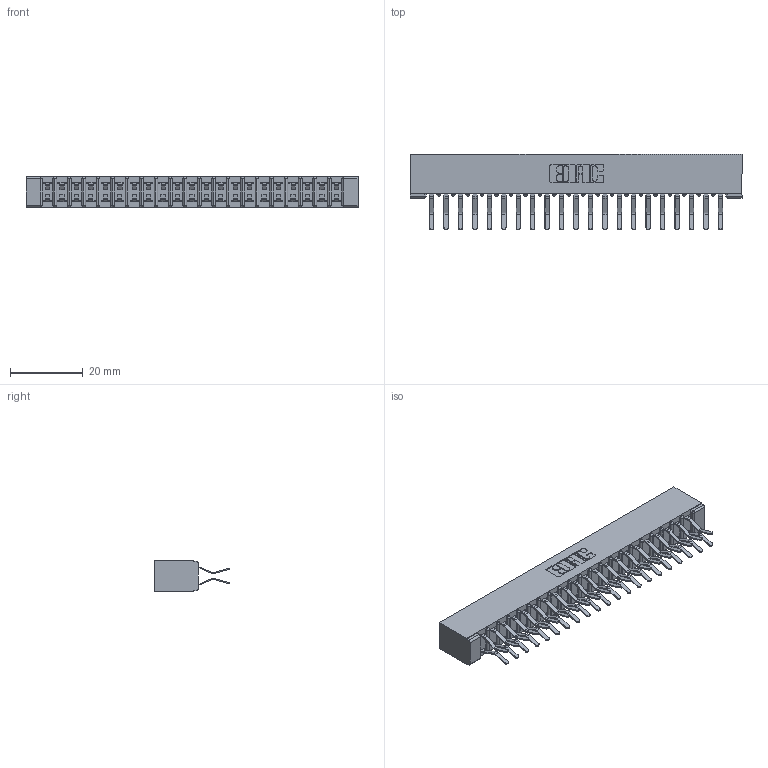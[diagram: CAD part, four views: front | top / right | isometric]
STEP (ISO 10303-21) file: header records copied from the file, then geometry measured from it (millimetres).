
FILE_DESCRIPTION (( 'STEP AP203' ), '1' );
FILE_NAME ('357-042-560-201.STEP', '2018-08-11T09:21:15', ( '' ), ( '' ), 'SwSTEP 2.0', 'SolidWorks 2016', '' );
FILE_SCHEMA (( 'CONFIG_CONTROL_DESIGN' ));
Length unit declared in the file: inch
Products named in the file (3): 307-290-001_560; 357-042-560-201; 307 Part_No Mounting Lugs
Assembly tree (43 placements, depth 2):
  357-042-560-201
    307 Part_No Mounting Lugs
    307-290-001_560  x42
Bounding box: 91.08 x 20.73 x 8.71 mm (x, y, z)
Volume: 6243.5 mm3; surface area: 11764 mm2
Topology: 43 solids, 43 shells, 2232 faces, 6263 edges, 4058 vertices
Faces by surface type: plane 1452, cylinder 736, sphere 44
Entity records: 21090 total; most frequent: CARTESIAN_POINT 3453, ORIENTED_EDGE 3418, DIRECTION 3391, EDGE_CURVE 1709, LINE 1303, VECTOR 1303, VERTEX_POINT 1106, AXIS2_PLACEMENT_3D 1044
